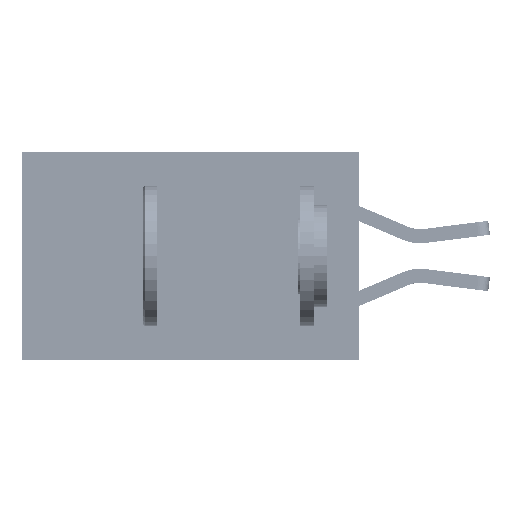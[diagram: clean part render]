
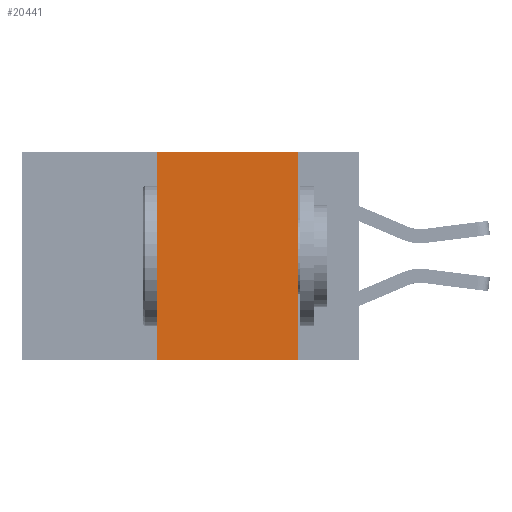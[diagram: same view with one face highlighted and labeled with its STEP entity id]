
A CAD part, left-side view. The second image highlights one B-rep face of the part: STEP entity #20441.
In plain terms, the highlighted planar face has unit normal (-1, 0, 0).
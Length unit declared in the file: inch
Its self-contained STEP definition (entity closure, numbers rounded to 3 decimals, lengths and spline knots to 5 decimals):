
#2553 = VECTOR ( 'NONE', #18657, 39.37008 ) ;
#5355 = EDGE_CURVE ( 'NONE', #19866, #18165, #38797, .T. ) ;
#8885 = ORIENTED_EDGE ( 'NONE', *, *, #32198, .F. ) ;
#10222 = CARTESIAN_POINT ( 'NONE',  ( 0., 0.6, 0. ) ) ;
#10617 = VECTOR ( 'NONE', #10671, 39.37008 ) ;
#10671 = DIRECTION ( 'NONE',  ( 0., 0., -1. ) ) ;
#11403 = CARTESIAN_POINT ( 'NONE',  ( 0., 0.6, -0.37 ) ) ;
#13460 = DIRECTION ( 'NONE',  ( 0., -1., 0. ) ) ;
#14824 = CARTESIAN_POINT ( 'NONE',  ( 0., 0.36, -0.37 ) ) ;
#15426 = CARTESIAN_POINT ( 'NONE',  ( 0., 0.36, 0. ) ) ;
#15871 = EDGE_CURVE ( 'NONE', #33291, #30121, #20414, .T. ) ;
#16198 = DIRECTION ( 'NONE',  ( 0., 0., -1. ) ) ;
#17690 = CARTESIAN_POINT ( 'NONE',  ( 0., 0.36, 0. ) ) ;
#18165 = VERTEX_POINT ( 'NONE', #31059 ) ;
#18657 = DIRECTION ( 'NONE',  ( 0., 0., 1. ) ) ;
#19497 = ORIENTED_EDGE ( 'NONE', *, *, #28707, .F. ) ;
#19866 = VERTEX_POINT ( 'NONE', #17690 ) ;
#20414 = LINE ( 'NONE', #11403, #36370 ) ;
#20441 = ADVANCED_FACE ( 'NONE', ( #34527 ), #28891, .F. ) ;
#21509 = ORIENTED_EDGE ( 'NONE', *, *, #15871, .T. ) ;
#22741 = CARTESIAN_POINT ( 'NONE',  ( 0., 0.11, -0.37 ) ) ;
#23462 = CARTESIAN_POINT ( 'NONE',  ( 0., 0.11, 0. ) ) ;
#25496 = AXIS2_PLACEMENT_3D ( 'NONE', #25727, #35317, #16198 ) ;
#25727 = CARTESIAN_POINT ( 'NONE',  ( 0., 0.6, 0. ) ) ;
#28378 = EDGE_LOOP ( 'NONE', ( #8885, #35450, #19497, #21509 ) ) ;
#28707 = EDGE_CURVE ( 'NONE', #33291, #19866, #37004, .T. ) ;
#28891 = PLANE ( 'NONE',  #25496 ) ;
#30121 = VERTEX_POINT ( 'NONE', #22741 ) ;
#30322 = VECTOR ( 'NONE', #13460, 39.37008 ) ;
#30589 = DIRECTION ( 'NONE',  ( 0., -1., 0. ) ) ;
#31059 = CARTESIAN_POINT ( 'NONE',  ( 0., 0.11, 0. ) ) ;
#32198 = EDGE_CURVE ( 'NONE', #18165, #30121, #36165, .T. ) ;
#33291 = VERTEX_POINT ( 'NONE', #14824 ) ;
#34527 = FACE_OUTER_BOUND ( 'NONE', #28378, .T. ) ;
#35317 = DIRECTION ( 'NONE',  ( 1., 0., 0. ) ) ;
#35450 = ORIENTED_EDGE ( 'NONE', *, *, #5355, .F. ) ;
#36165 = LINE ( 'NONE', #23462, #10617 ) ;
#36370 = VECTOR ( 'NONE', #30589, 39.37008 ) ;
#37004 = LINE ( 'NONE', #15426, #2553 ) ;
#38797 = LINE ( 'NONE', #10222, #30322 ) ;
